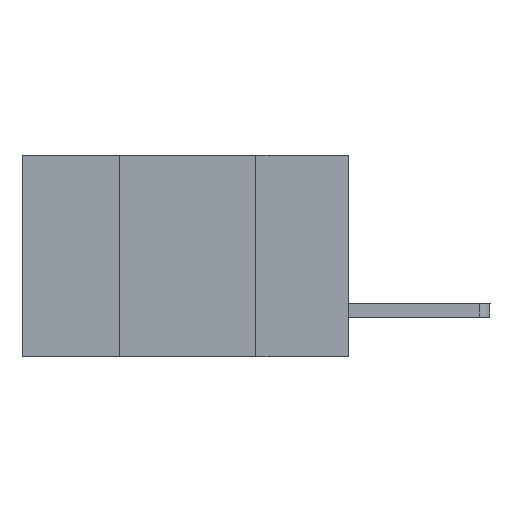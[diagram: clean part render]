
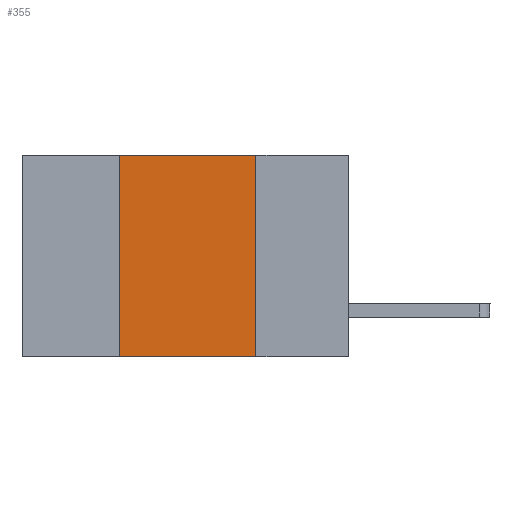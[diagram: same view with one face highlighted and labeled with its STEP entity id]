
A CAD part, left-side view. The second image highlights one B-rep face of the part: STEP entity #355.
In plain terms, the highlighted planar face has unit normal (-1, 0, 0).
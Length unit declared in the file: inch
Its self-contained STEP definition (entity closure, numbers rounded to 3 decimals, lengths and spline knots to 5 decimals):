
#355 = ADVANCED_FACE ( 'NONE', ( #4306 ), #3079, .F. ) ;
#392 = DIRECTION ( 'NONE',  ( 0., 0., -1. ) ) ;
#705 = VECTOR ( 'NONE', #4010, 39.37008 ) ;
#1086 = VECTOR ( 'NONE', #7279, 39.37008 ) ;
#1152 = CARTESIAN_POINT ( 'NONE',  ( 0., 0.17, 0. ) ) ;
#1185 = VERTEX_POINT ( 'NONE', #1152 ) ;
#2347 = CARTESIAN_POINT ( 'NONE',  ( 0., 0.17, -0.37 ) ) ;
#2598 = VERTEX_POINT ( 'NONE', #5230 ) ;
#2824 = CARTESIAN_POINT ( 'NONE',  ( 0., 0.6, -0.37 ) ) ;
#3079 = PLANE ( 'NONE',  #6440 ) ;
#3172 = ORIENTED_EDGE ( 'NONE', *, *, #6951, .F. ) ;
#3240 = LINE ( 'NONE', #3296, #8286 ) ;
#3296 = CARTESIAN_POINT ( 'NONE',  ( 0., 0.6, 0. ) ) ;
#3318 = EDGE_CURVE ( 'NONE', #2598, #1185, #3240, .T. ) ;
#3504 = VERTEX_POINT ( 'NONE', #5333 ) ;
#3802 = DIRECTION ( 'NONE',  ( 0., 0., -1. ) ) ;
#4010 = DIRECTION ( 'NONE',  ( 0., -1., 0. ) ) ;
#4306 = FACE_OUTER_BOUND ( 'NONE', #8084, .T. ) ;
#4561 = DIRECTION ( 'NONE',  ( 0., -1., 0. ) ) ;
#4730 = ORIENTED_EDGE ( 'NONE', *, *, #7894, .T. ) ;
#5230 = CARTESIAN_POINT ( 'NONE',  ( 0., 0.42, 0. ) ) ;
#5333 = CARTESIAN_POINT ( 'NONE',  ( 0., 0.17, -0.37 ) ) ;
#5724 = ORIENTED_EDGE ( 'NONE', *, *, #8394, .F. ) ;
#5856 = VECTOR ( 'NONE', #392, 39.37008 ) ;
#6253 = LINE ( 'NONE', #2347, #5856 ) ;
#6440 = AXIS2_PLACEMENT_3D ( 'NONE', #6900, #6856, #3802 ) ;
#6681 = CARTESIAN_POINT ( 'NONE',  ( 0., 0.42, -0.37 ) ) ;
#6856 = DIRECTION ( 'NONE',  ( 1., 0., 0. ) ) ;
#6900 = CARTESIAN_POINT ( 'NONE',  ( 0., 0.6, 0. ) ) ;
#6951 = EDGE_CURVE ( 'NONE', #7017, #2598, #7314, .T. ) ;
#7017 = VERTEX_POINT ( 'NONE', #7875 ) ;
#7106 = ORIENTED_EDGE ( 'NONE', *, *, #3318, .F. ) ;
#7279 = DIRECTION ( 'NONE',  ( 0., 0., 1. ) ) ;
#7314 = LINE ( 'NONE', #6681, #1086 ) ;
#7875 = CARTESIAN_POINT ( 'NONE',  ( 0., 0.42, -0.37 ) ) ;
#7894 = EDGE_CURVE ( 'NONE', #7017, #3504, #8052, .T. ) ;
#8052 = LINE ( 'NONE', #2824, #705 ) ;
#8084 = EDGE_LOOP ( 'NONE', ( #5724, #7106, #3172, #4730 ) ) ;
#8286 = VECTOR ( 'NONE', #4561, 39.37008 ) ;
#8394 = EDGE_CURVE ( 'NONE', #1185, #3504, #6253, .T. ) ;
